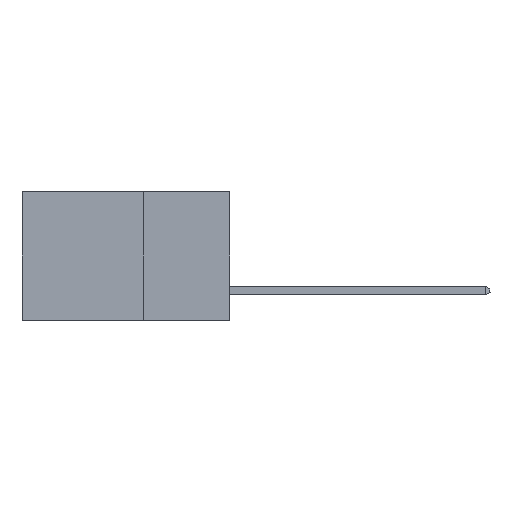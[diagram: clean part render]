
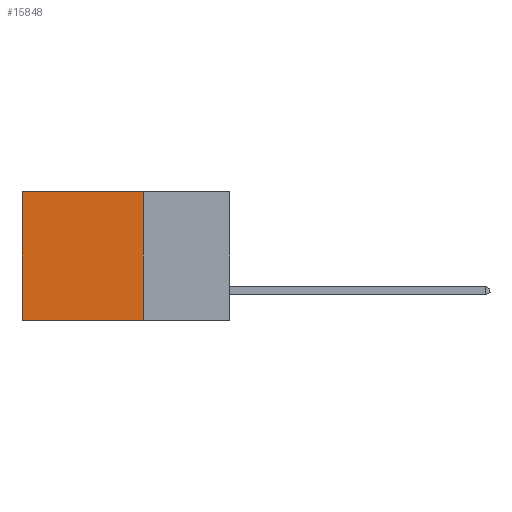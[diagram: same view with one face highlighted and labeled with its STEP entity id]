
A CAD part, left-side view. The second image highlights one B-rep face of the part: STEP entity #15848.
In plain terms, the highlighted planar face has unit normal (-1, 0, 0).
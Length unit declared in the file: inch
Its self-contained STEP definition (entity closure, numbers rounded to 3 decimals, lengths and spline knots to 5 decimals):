
#106 = CARTESIAN_POINT ( 'NONE',  ( 0.298, 0.25, 0. ) ) ;
#127 = CARTESIAN_POINT ( 'NONE',  ( 0.298, 0.25, 0. ) ) ;
#1615 = CARTESIAN_POINT ( 'NONE',  ( 0.298, 0.6, 0. ) ) ;
#1795 = CARTESIAN_POINT ( 'NONE',  ( 0.298, 0.25, -0.37 ) ) ;
#2062 = VERTEX_POINT ( 'NONE', #18572 ) ;
#3777 = VECTOR ( 'NONE', #3827, 39.37008 ) ;
#3827 = DIRECTION ( 'NONE',  ( 0., 1., 0. ) ) ;
#3846 = ORIENTED_EDGE ( 'NONE', *, *, #13557, .T. ) ;
#4218 = VERTEX_POINT ( 'NONE', #106 ) ;
#5448 = ORIENTED_EDGE ( 'NONE', *, *, #18086, .T. ) ;
#5997 = CARTESIAN_POINT ( 'NONE',  ( 0.298, 0.25, 0. ) ) ;
#7009 = LINE ( 'NONE', #17778, #11879 ) ;
#7360 = EDGE_LOOP ( 'NONE', ( #3846, #13166, #18522, #5448 ) ) ;
#8999 = DIRECTION ( 'NONE',  ( 0., 1., 0. ) ) ;
#9107 = AXIS2_PLACEMENT_3D ( 'NONE', #5997, #13403, #14738 ) ;
#9611 = DIRECTION ( 'NONE',  ( 0., 0., -1. ) ) ;
#9928 = VECTOR ( 'NONE', #9611, 39.37008 ) ;
#11573 = LINE ( 'NONE', #1795, #3777 ) ;
#11879 = VECTOR ( 'NONE', #8999, 39.37008 ) ;
#12236 = CARTESIAN_POINT ( 'NONE',  ( 0.298, 0.6, 0. ) ) ;
#12518 = EDGE_CURVE ( 'NONE', #4218, #17338, #12600, .T. ) ;
#12600 = LINE ( 'NONE', #127, #16943 ) ;
#13166 = ORIENTED_EDGE ( 'NONE', *, *, #13400, .F. ) ;
#13179 = LINE ( 'NONE', #12236, #9928 ) ;
#13239 = DIRECTION ( 'NONE',  ( 0., 0., -1. ) ) ;
#13400 = EDGE_CURVE ( 'NONE', #17338, #2062, #11573, .T. ) ;
#13403 = DIRECTION ( 'NONE',  ( 1., 0., 0. ) ) ;
#13557 = EDGE_CURVE ( 'NONE', #14226, #2062, #13179, .T. ) ;
#13582 = PLANE ( 'NONE',  #9107 ) ;
#14226 = VERTEX_POINT ( 'NONE', #1615 ) ;
#14738 = DIRECTION ( 'NONE',  ( 0., 0., -1. ) ) ;
#15848 = ADVANCED_FACE ( 'NONE', ( #16313 ), #13582, .F. ) ;
#16313 = FACE_OUTER_BOUND ( 'NONE', #7360, .T. ) ;
#16943 = VECTOR ( 'NONE', #13239, 39.37008 ) ;
#17338 = VERTEX_POINT ( 'NONE', #18541 ) ;
#17778 = CARTESIAN_POINT ( 'NONE',  ( 0.298, 0.25, 0. ) ) ;
#18086 = EDGE_CURVE ( 'NONE', #4218, #14226, #7009, .T. ) ;
#18522 = ORIENTED_EDGE ( 'NONE', *, *, #12518, .F. ) ;
#18541 = CARTESIAN_POINT ( 'NONE',  ( 0.298, 0.25, -0.37 ) ) ;
#18572 = CARTESIAN_POINT ( 'NONE',  ( 0.298, 0.6, -0.37 ) ) ;
